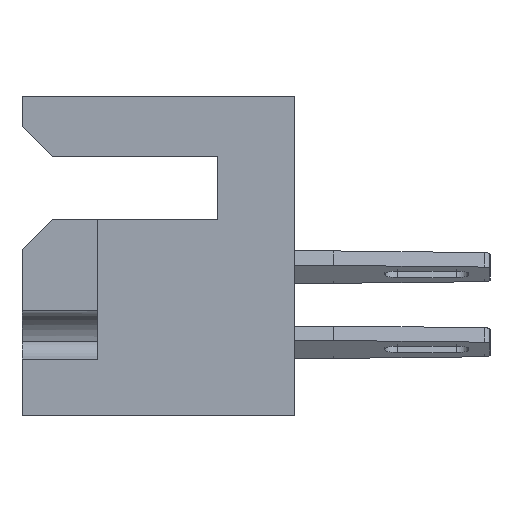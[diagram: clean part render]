
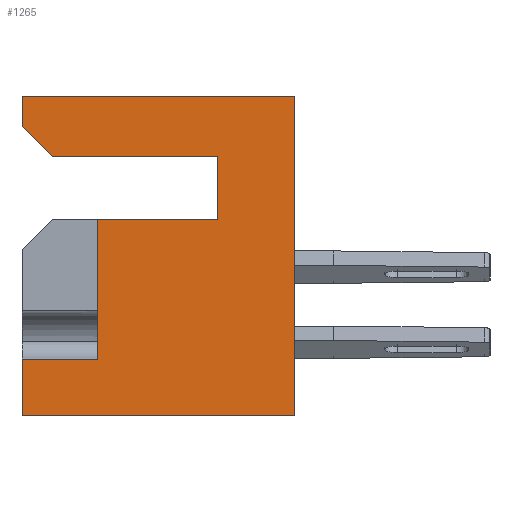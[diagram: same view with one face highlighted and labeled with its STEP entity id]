
A CAD part, left-side view. The second image highlights one B-rep face of the part: STEP entity #1265.
In plain terms, the highlighted planar face has unit normal (-1, 0, 0).
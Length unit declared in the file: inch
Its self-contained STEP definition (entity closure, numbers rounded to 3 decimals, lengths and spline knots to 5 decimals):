
#766 = DIRECTION ( 'NONE',  ( 0., 1., 0. ) ) ;
#1126 = LINE ( 'NONE', #14037, #3116 ) ;
#1265 = ADVANCED_FACE ( 'NONE', ( #9525 ), #10728, .F. ) ;
#2611 = EDGE_CURVE ( 'NONE', #7337, #4344, #19973, .T. ) ;
#3036 = LINE ( 'NONE', #17407, #23167 ) ;
#3116 = VECTOR ( 'NONE', #5324, 39.37008 ) ;
#3193 = DIRECTION ( 'NONE',  ( 0., 0., 1. ) ) ;
#3870 = DIRECTION ( 'NONE',  ( 0., -0.707, -0.707 ) ) ;
#4176 = CARTESIAN_POINT ( 'NONE',  ( 0., 0.328, -0.205 ) ) ;
#4224 = LINE ( 'NONE', #17742, #10840 ) ;
#4237 = DIRECTION ( 'NONE',  ( 0., 0., -1. ) ) ;
#4304 = LINE ( 'NONE', #19887, #10916 ) ;
#4344 = VERTEX_POINT ( 'NONE', #5476 ) ;
#4443 = VECTOR ( 'NONE', #7560, 39.37008 ) ;
#5324 = DIRECTION ( 'NONE',  ( 0., 0., 1. ) ) ;
#5381 = ORIENTED_EDGE ( 'NONE', *, *, #20708, .F. ) ;
#5476 = CARTESIAN_POINT ( 'NONE',  ( 0., 0.403, -0.1 ) ) ;
#5576 = VECTOR ( 'NONE', #766, 39.37008 ) ;
#6381 = CARTESIAN_POINT ( 'NONE',  ( 0., 0.453, 0. ) ) ;
#6434 = VERTEX_POINT ( 'NONE', #14225 ) ;
#6483 = VECTOR ( 'NONE', #3870, 39.37008 ) ;
#7278 = LINE ( 'NONE', #13444, #5576 ) ;
#7337 = VERTEX_POINT ( 'NONE', #12803 ) ;
#7560 = DIRECTION ( 'NONE',  ( 0., 0., 1. ) ) ;
#7865 = DIRECTION ( 'NONE',  ( 0., -1., 0. ) ) ;
#9000 = EDGE_CURVE ( 'NONE', #12957, #24624, #22260, .T. ) ;
#9231 = EDGE_CURVE ( 'NONE', #25901, #4344, #26565, .T. ) ;
#9476 = DIRECTION ( 'NONE',  ( 0., 0., 1. ) ) ;
#9525 = FACE_OUTER_BOUND ( 'NONE', #23055, .T. ) ;
#9609 = EDGE_CURVE ( 'NONE', #12320, #24624, #16966, .T. ) ;
#9684 = ORIENTED_EDGE ( 'NONE', *, *, #23152, .F. ) ;
#9970 = CARTESIAN_POINT ( 'NONE',  ( 0., 0., 0. ) ) ;
#10706 = VERTEX_POINT ( 'NONE', #4176 ) ;
#10716 = VECTOR ( 'NONE', #14666, 39.37008 ) ;
#10728 = PLANE ( 'NONE',  #16467 ) ;
#10816 = VECTOR ( 'NONE', #7865, 39.37008 ) ;
#10840 = VECTOR ( 'NONE', #3193, 39.37008 ) ;
#10848 = CARTESIAN_POINT ( 'NONE',  ( 0., 0.453, -0.437 ) ) ;
#10916 = VECTOR ( 'NONE', #9476, 39.37008 ) ;
#11631 = ORIENTED_EDGE ( 'NONE', *, *, #9609, .F. ) ;
#11676 = ORIENTED_EDGE ( 'NONE', *, *, #2611, .T. ) ;
#11677 = CARTESIAN_POINT ( 'NONE',  ( 0., 0.128, -0.1 ) ) ;
#11901 = CARTESIAN_POINT ( 'NONE',  ( 0., 0.128, -0.205 ) ) ;
#12037 = CARTESIAN_POINT ( 'NONE',  ( 0., 0.128, -0.205 ) ) ;
#12210 = CARTESIAN_POINT ( 'NONE',  ( 0., 0.453, 0. ) ) ;
#12320 = VERTEX_POINT ( 'NONE', #12210 ) ;
#12682 = ORIENTED_EDGE ( 'NONE', *, *, #14954, .F. ) ;
#12803 = CARTESIAN_POINT ( 'NONE',  ( 0., 0.453, -0.05 ) ) ;
#12861 = VERTEX_POINT ( 'NONE', #17598 ) ;
#12957 = VERTEX_POINT ( 'NONE', #13751 ) ;
#13444 = CARTESIAN_POINT ( 'NONE',  ( 0., 0.328, -0.437 ) ) ;
#13751 = CARTESIAN_POINT ( 'NONE',  ( 0., 0., -0.531 ) ) ;
#13788 = EDGE_CURVE ( 'NONE', #15840, #10706, #19311, .T. ) ;
#13816 = DIRECTION ( 'NONE',  ( 0., 0., 1. ) ) ;
#13968 = ORIENTED_EDGE ( 'NONE', *, *, #13788, .T. ) ;
#14037 = CARTESIAN_POINT ( 'NONE',  ( 0., 0.128, -0.1 ) ) ;
#14225 = CARTESIAN_POINT ( 'NONE',  ( 0., 0.453, -0.531 ) ) ;
#14345 = VECTOR ( 'NONE', #22020, 39.37008 ) ;
#14666 = DIRECTION ( 'NONE',  ( 0., 1., 0. ) ) ;
#14954 = EDGE_CURVE ( 'NONE', #15840, #25901, #1126, .T. ) ;
#15840 = VERTEX_POINT ( 'NONE', #11901 ) ;
#16072 = LINE ( 'NONE', #16438, #10816 ) ;
#16438 = CARTESIAN_POINT ( 'NONE',  ( 0., 0.453, -0.531 ) ) ;
#16467 = AXIS2_PLACEMENT_3D ( 'NONE', #6381, #21393, #4237 ) ;
#16522 = CARTESIAN_POINT ( 'NONE',  ( 0., 0.403, -0.1 ) ) ;
#16966 = LINE ( 'NONE', #19892, #14345 ) ;
#17407 = CARTESIAN_POINT ( 'NONE',  ( 0., 0.328, -0.205 ) ) ;
#17598 = CARTESIAN_POINT ( 'NONE',  ( 0., 0.328, -0.437 ) ) ;
#17742 = CARTESIAN_POINT ( 'NONE',  ( 0., 0.453, 0. ) ) ;
#18556 = DIRECTION ( 'NONE',  ( 0., 1., 0. ) ) ;
#18908 = ORIENTED_EDGE ( 'NONE', *, *, #25956, .T. ) ;
#19311 = LINE ( 'NONE', #12037, #26948 ) ;
#19887 = CARTESIAN_POINT ( 'NONE',  ( 0., 0.453, 0. ) ) ;
#19892 = CARTESIAN_POINT ( 'NONE',  ( 0., 0.453, 0. ) ) ;
#19973 = LINE ( 'NONE', #16522, #6483 ) ;
#20708 = EDGE_CURVE ( 'NONE', #6434, #25540, #4304, .T. ) ;
#20882 = ORIENTED_EDGE ( 'NONE', *, *, #9231, .F. ) ;
#21393 = DIRECTION ( 'NONE',  ( 1., 0., 0. ) ) ;
#21965 = EDGE_CURVE ( 'NONE', #12861, #25540, #7278, .T. ) ;
#22020 = DIRECTION ( 'NONE',  ( 0., -1., 0. ) ) ;
#22260 = LINE ( 'NONE', #26478, #4443 ) ;
#22598 = ORIENTED_EDGE ( 'NONE', *, *, #9000, .T. ) ;
#23055 = EDGE_LOOP ( 'NONE', ( #25711, #5381, #18908, #22598, #11631, #23457, #11676, #20882, #12682, #13968, #9684 ) ) ;
#23152 = EDGE_CURVE ( 'NONE', #12861, #10706, #3036, .T. ) ;
#23167 = VECTOR ( 'NONE', #13816, 39.37008 ) ;
#23457 = ORIENTED_EDGE ( 'NONE', *, *, #25188, .F. ) ;
#24624 = VERTEX_POINT ( 'NONE', #9970 ) ;
#25188 = EDGE_CURVE ( 'NONE', #7337, #12320, #4224, .T. ) ;
#25540 = VERTEX_POINT ( 'NONE', #10848 ) ;
#25711 = ORIENTED_EDGE ( 'NONE', *, *, #21965, .T. ) ;
#25901 = VERTEX_POINT ( 'NONE', #11677 ) ;
#25956 = EDGE_CURVE ( 'NONE', #6434, #12957, #16072, .T. ) ;
#26478 = CARTESIAN_POINT ( 'NONE',  ( 0., 0., 0. ) ) ;
#26565 = LINE ( 'NONE', #27108, #10716 ) ;
#26948 = VECTOR ( 'NONE', #18556, 39.37008 ) ;
#27108 = CARTESIAN_POINT ( 'NONE',  ( 0., 0.128, -0.1 ) ) ;
